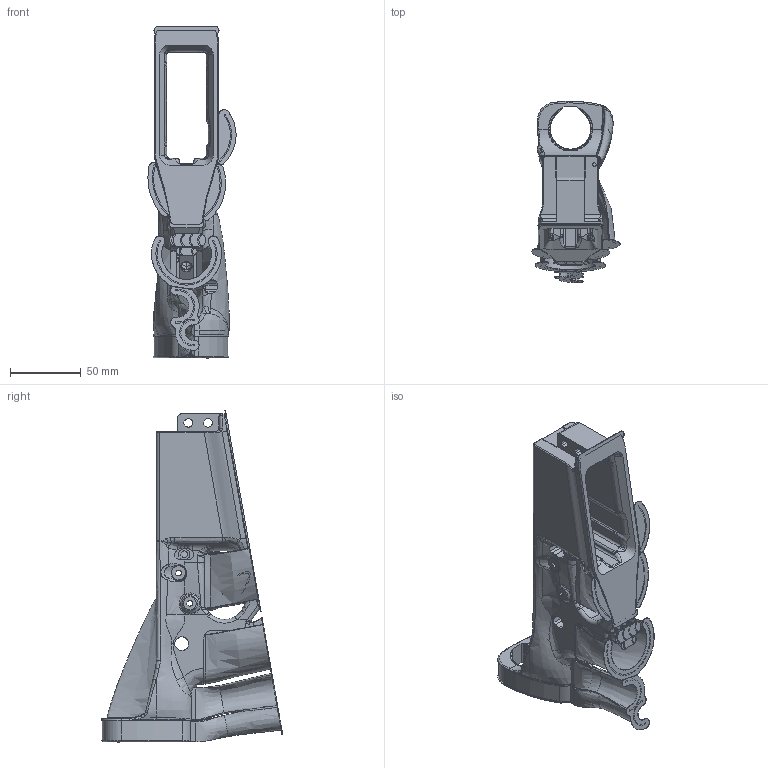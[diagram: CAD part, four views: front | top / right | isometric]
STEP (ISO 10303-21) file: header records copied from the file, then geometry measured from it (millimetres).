
FILE_DESCRIPTION (( 'STEP AP203' ), '1' );
FILE_NAME ('LR-308 SL V2.6.STEP', '2022-05-15T12:46:38', ( '' ), ( '' ), 'SwSTEP 2.0', 'SolidWorks 2021', '' );
FILE_SCHEMA (( 'CONFIG_CONTROL_DESIGN' ));
Products named in the file (1): LR-308 SL V2.6
Bounding box: 62.42 x 128.11 x 234.71 mm (x, y, z)
Volume: 219547.4 mm3; surface area: 113457.5 mm2
Topology: 8 solids, 8 shells, 2163 faces, 6027 edges, 3909 vertices
Faces by surface type: bspline 1033, plane 635, cylinder 400, torus 61, cone 24, sphere 10
Entity records: 235501 total; most frequent: CARTESIAN_POINT 188713, ORIENTED_EDGE 11936, DIRECTION 6344, EDGE_CURVE 5968, VERTEX_POINT 3909, B_SPLINE_CURVE_WITH_KNOTS 2483, LINE 2338, VECTOR 2338
